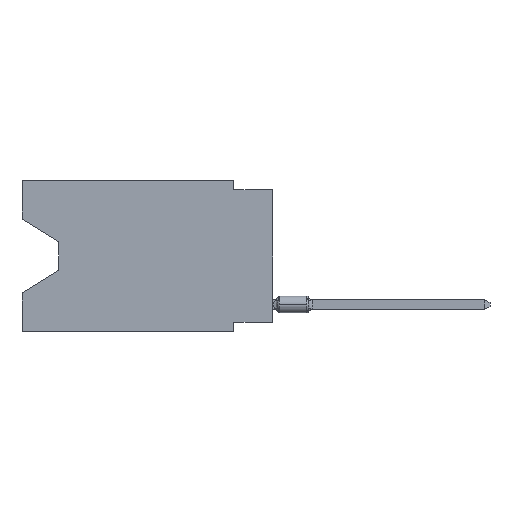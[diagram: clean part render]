
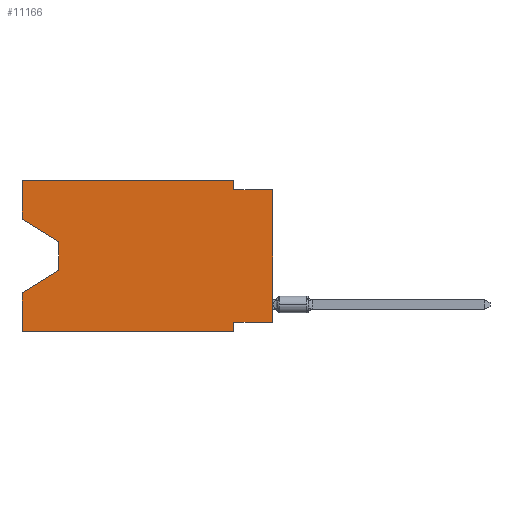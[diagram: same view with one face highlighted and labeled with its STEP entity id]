
A CAD part, left-side view. The second image highlights one B-rep face of the part: STEP entity #11166.
In plain terms, the highlighted planar face has unit normal (-1, 0, 0).
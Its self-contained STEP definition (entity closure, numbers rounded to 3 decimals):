
#295 = VERTEX_POINT ( 'NONE', #10167 ) ;
#542 = EDGE_CURVE ( 'NONE', #6794, #3437, #9859, .T. ) ;
#897 = LINE ( 'NONE', #5289, #10562 ) ;
#1003 = CARTESIAN_POINT ( 'NONE',  ( 0., 2.54, 0. ) ) ;
#1004 = CARTESIAN_POINT ( 'NONE',  ( 0., 16.383, -7.36 ) ) ;
#1020 = LINE ( 'NONE', #12081, #5798 ) ;
#1051 = DIRECTION ( 'NONE',  ( 0., 0., 1. ) ) ;
#1095 = CARTESIAN_POINT ( 'NONE',  ( 0., 13.97, -5.893 ) ) ;
#1168 = DIRECTION ( 'NONE',  ( 1., 0., 0. ) ) ;
#1247 = VERTEX_POINT ( 'NONE', #6160 ) ;
#1260 = VECTOR ( 'NONE', #9641, 1000. ) ;
#1605 = VECTOR ( 'NONE', #4082, 1000. ) ;
#1699 = LINE ( 'NONE', #2939, #10477 ) ;
#1832 = AXIS2_PLACEMENT_3D ( 'NONE', #13155, #1168, #3113 ) ;
#1850 = LINE ( 'NONE', #13896, #1605 ) ;
#1994 = EDGE_CURVE ( 'NONE', #13931, #6794, #8270, .T. ) ;
#2170 = EDGE_CURVE ( 'NONE', #13500, #1247, #1699, .T. ) ;
#2791 = ORIENTED_EDGE ( 'NONE', *, *, #2170, .F. ) ;
#2939 = CARTESIAN_POINT ( 'NONE',  ( 0., 0., -9.271 ) ) ;
#3008 = DIRECTION ( 'NONE',  ( 0., 1., 0. ) ) ;
#3113 = DIRECTION ( 'NONE',  ( 0., 0., -1. ) ) ;
#3205 = CARTESIAN_POINT ( 'NONE',  ( 0., 2.54, -9.906 ) ) ;
#3291 = LINE ( 'NONE', #11970, #11482 ) ;
#3437 = VERTEX_POINT ( 'NONE', #1004 ) ;
#3620 = DIRECTION ( 'NONE',  ( 0., -1., 0. ) ) ;
#3818 = ORIENTED_EDGE ( 'NONE', *, *, #8345, .F. ) ;
#4082 = DIRECTION ( 'NONE',  ( 0., 0., -1. ) ) ;
#4106 = CARTESIAN_POINT ( 'NONE',  ( 0., 16.383, -9.906 ) ) ;
#4155 = EDGE_CURVE ( 'NONE', #10563, #10177, #13918, .T. ) ;
#4425 = ORIENTED_EDGE ( 'NONE', *, *, #9869, .F. ) ;
#4436 = CARTESIAN_POINT ( 'NONE',  ( 0., 13.97, -4.013 ) ) ;
#5289 = CARTESIAN_POINT ( 'NONE',  ( 0., 0., 0. ) ) ;
#5363 = ORIENTED_EDGE ( 'NONE', *, *, #7290, .F. ) ;
#5426 = ORIENTED_EDGE ( 'NONE', *, *, #6793, .T. ) ;
#5453 = LINE ( 'NONE', #5525, #5933 ) ;
#5525 = CARTESIAN_POINT ( 'NONE',  ( 0., 16.383, 0. ) ) ;
#5798 = VECTOR ( 'NONE', #13159, 1000. ) ;
#5933 = VECTOR ( 'NONE', #9832, 1000. ) ;
#5938 = ORIENTED_EDGE ( 'NONE', *, *, #10840, .F. ) ;
#6160 = CARTESIAN_POINT ( 'NONE',  ( 0., 2.54, -9.271 ) ) ;
#6353 = LINE ( 'NONE', #3205, #7114 ) ;
#6519 = ORIENTED_EDGE ( 'NONE', *, *, #9810, .F. ) ;
#6793 = EDGE_CURVE ( 'NONE', #13500, #12141, #897, .T. ) ;
#6794 = VERTEX_POINT ( 'NONE', #14027 ) ;
#6866 = EDGE_LOOP ( 'NONE', ( #10132, #9580, #12074, #3818, #8435, #5938, #2791, #5426, #10938, #6519, #5363, #4425 ) ) ;
#6918 = LINE ( 'NONE', #11295, #10146 ) ;
#6952 = CARTESIAN_POINT ( 'NONE',  ( 0., 16.383, -2.546 ) ) ;
#7114 = VECTOR ( 'NONE', #10734, 1000. ) ;
#7290 = EDGE_CURVE ( 'NONE', #295, #12910, #6918, .T. ) ;
#7549 = LINE ( 'NONE', #9854, #13120 ) ;
#8270 = LINE ( 'NONE', #12638, #12292 ) ;
#8345 = EDGE_CURVE ( 'NONE', #10563, #3437, #5453, .T. ) ;
#8435 = ORIENTED_EDGE ( 'NONE', *, *, #4155, .T. ) ;
#8441 = VECTOR ( 'NONE', #8475, 1000. ) ;
#8475 = DIRECTION ( 'NONE',  ( 0., -1., 0. ) ) ;
#9580 = ORIENTED_EDGE ( 'NONE', *, *, #1994, .T. ) ;
#9592 = VERTEX_POINT ( 'NONE', #6952 ) ;
#9635 = DIRECTION ( 'NONE',  ( 0., -1., 0. ) ) ;
#9641 = DIRECTION ( 'NONE',  ( 0., 0.855, -0.519 ) ) ;
#9666 = DIRECTION ( 'NONE',  ( 0., 0., 1. ) ) ;
#9729 = VERTEX_POINT ( 'NONE', #14103 ) ;
#9810 = EDGE_CURVE ( 'NONE', #12910, #9729, #1850, .T. ) ;
#9832 = DIRECTION ( 'NONE',  ( 0., 0., 1. ) ) ;
#9854 = CARTESIAN_POINT ( 'NONE',  ( 0., 0., -0.635 ) ) ;
#9858 = PLANE ( 'NONE',  #1832 ) ;
#9859 = LINE ( 'NONE', #1095, #1260 ) ;
#9869 = EDGE_CURVE ( 'NONE', #9592, #295, #3291, .T. ) ;
#10132 = ORIENTED_EDGE ( 'NONE', *, *, #12498, .T. ) ;
#10146 = VECTOR ( 'NONE', #3620, 1000. ) ;
#10167 = CARTESIAN_POINT ( 'NONE',  ( 0., 16.383, 0. ) ) ;
#10177 = VERTEX_POINT ( 'NONE', #13572 ) ;
#10477 = VECTOR ( 'NONE', #3008, 1000. ) ;
#10562 = VECTOR ( 'NONE', #9666, 1000. ) ;
#10563 = VERTEX_POINT ( 'NONE', #13342 ) ;
#10734 = DIRECTION ( 'NONE',  ( 0., 0., -1. ) ) ;
#10840 = EDGE_CURVE ( 'NONE', #1247, #10177, #6353, .T. ) ;
#10938 = ORIENTED_EDGE ( 'NONE', *, *, #11845, .F. ) ;
#11166 = ADVANCED_FACE ( 'NONE', ( #13798 ), #9858, .F. ) ;
#11295 = CARTESIAN_POINT ( 'NONE',  ( 0., 16.383, 0. ) ) ;
#11482 = VECTOR ( 'NONE', #1051, 1000. ) ;
#11505 = DIRECTION ( 'NONE',  ( 0., 0., -1. ) ) ;
#11845 = EDGE_CURVE ( 'NONE', #9729, #12141, #7549, .T. ) ;
#11970 = CARTESIAN_POINT ( 'NONE',  ( 0., 16.383, 0. ) ) ;
#12074 = ORIENTED_EDGE ( 'NONE', *, *, #542, .T. ) ;
#12081 = CARTESIAN_POINT ( 'NONE',  ( 0., 16.383, -2.546 ) ) ;
#12141 = VERTEX_POINT ( 'NONE', #12170 ) ;
#12170 = CARTESIAN_POINT ( 'NONE',  ( 0., 0., -0.635 ) ) ;
#12292 = VECTOR ( 'NONE', #11505, 1000. ) ;
#12498 = EDGE_CURVE ( 'NONE', #9592, #13931, #1020, .T. ) ;
#12638 = CARTESIAN_POINT ( 'NONE',  ( 0., 13.97, -4.013 ) ) ;
#12910 = VERTEX_POINT ( 'NONE', #1003 ) ;
#13120 = VECTOR ( 'NONE', #9635, 1000. ) ;
#13155 = CARTESIAN_POINT ( 'NONE',  ( 0., 16.383, 0. ) ) ;
#13159 = DIRECTION ( 'NONE',  ( 0., -0.855, -0.519 ) ) ;
#13342 = CARTESIAN_POINT ( 'NONE',  ( 0., 16.383, -9.906 ) ) ;
#13500 = VERTEX_POINT ( 'NONE', #13642 ) ;
#13572 = CARTESIAN_POINT ( 'NONE',  ( 0., 2.54, -9.906 ) ) ;
#13642 = CARTESIAN_POINT ( 'NONE',  ( 0., 0., -9.271 ) ) ;
#13798 = FACE_OUTER_BOUND ( 'NONE', #6866, .T. ) ;
#13896 = CARTESIAN_POINT ( 'NONE',  ( 0., 2.54, 0. ) ) ;
#13918 = LINE ( 'NONE', #4106, #8441 ) ;
#13931 = VERTEX_POINT ( 'NONE', #4436 ) ;
#14027 = CARTESIAN_POINT ( 'NONE',  ( 0., 13.97, -5.893 ) ) ;
#14103 = CARTESIAN_POINT ( 'NONE',  ( 0., 2.54, -0.635 ) ) ;
